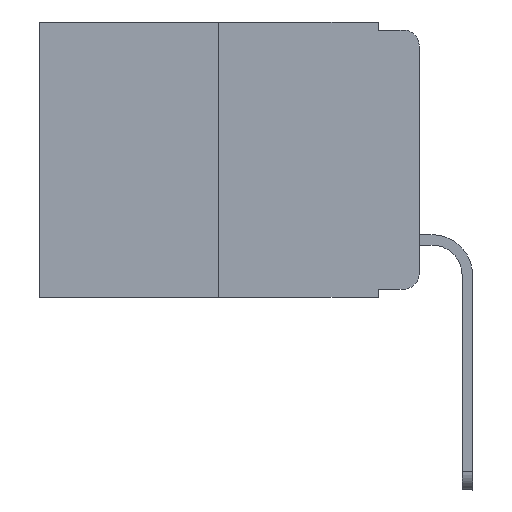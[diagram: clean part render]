
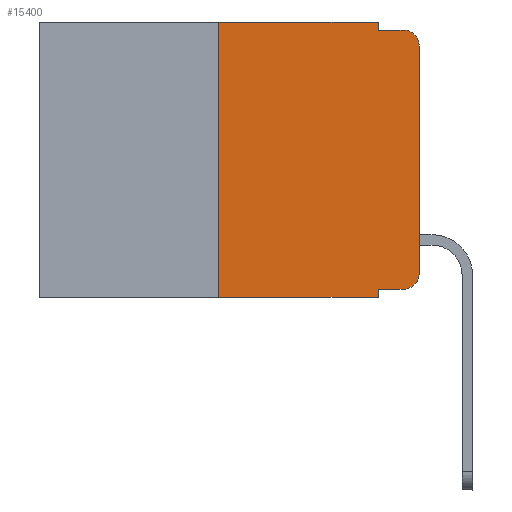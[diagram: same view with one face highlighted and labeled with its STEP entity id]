
A CAD part, left-side view. The second image highlights one B-rep face of the part: STEP entity #15400.
In plain terms, the highlighted planar face has unit normal (-1, 0, 0).
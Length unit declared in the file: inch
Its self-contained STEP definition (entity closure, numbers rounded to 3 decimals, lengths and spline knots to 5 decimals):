
#165 = VECTOR ( 'NONE', #6464, 39.37008 ) ;
#304 = EDGE_LOOP ( 'NONE', ( #10925, #14174, #7361, #12299, #2392, #10569, #844, #1517, #14218, #10826 ) ) ;
#573 = DIRECTION ( 'NONE',  ( 0., 0., 1. ) ) ;
#844 = ORIENTED_EDGE ( 'NONE', *, *, #16869, .T. ) ;
#1435 = CARTESIAN_POINT ( 'NONE',  ( 0., 0.051, 0. ) ) ;
#1517 = ORIENTED_EDGE ( 'NONE', *, *, #4754, .F. ) ;
#1707 = VECTOR ( 'NONE', #4496, 39.37008 ) ;
#1710 = DIRECTION ( 'NONE',  ( 1., 0., 0. ) ) ;
#2016 = LINE ( 'NONE', #16349, #14856 ) ;
#2392 = ORIENTED_EDGE ( 'NONE', *, *, #8061, .F. ) ;
#2592 = CARTESIAN_POINT ( 'NONE',  ( 0., 0.051, -0.01 ) ) ;
#2622 = LINE ( 'NONE', #18844, #1707 ) ;
#2809 = LINE ( 'NONE', #1435, #8584 ) ;
#2810 = CARTESIAN_POINT ( 'NONE',  ( 0., 0., -0.03 ) ) ;
#2931 = EDGE_CURVE ( 'NONE', #12350, #9406, #2622, .T. ) ;
#3103 = CIRCLE ( 'NONE', #6431, 0.02 ) ;
#3106 = CARTESIAN_POINT ( 'NONE',  ( 0., 0.051, -0.01 ) ) ;
#3170 = FACE_OUTER_BOUND ( 'NONE', #304, .T. ) ;
#3199 = VERTEX_POINT ( 'NONE', #14746 ) ;
#3351 = EDGE_CURVE ( 'NONE', #9406, #5729, #4566, .T. ) ;
#3366 = VERTEX_POINT ( 'NONE', #17032 ) ;
#3493 = CIRCLE ( 'NONE', #6182, 0.02 ) ;
#4496 = DIRECTION ( 'NONE',  ( 0., 0., -1. ) ) ;
#4566 = LINE ( 'NONE', #2592, #20115 ) ;
#4746 = LINE ( 'NONE', #6023, #20520 ) ;
#4754 = EDGE_CURVE ( 'NONE', #14351, #3199, #2809, .T. ) ;
#5729 = VERTEX_POINT ( 'NONE', #17383 ) ;
#5886 = DIRECTION ( 'NONE',  ( -1., 0., 0. ) ) ;
#6023 = CARTESIAN_POINT ( 'NONE',  ( 0., 0., 0. ) ) ;
#6074 = CARTESIAN_POINT ( 'NONE',  ( 0., 0.051, -0.333 ) ) ;
#6182 = AXIS2_PLACEMENT_3D ( 'NONE', #20226, #5886, #12489 ) ;
#6431 = AXIS2_PLACEMENT_3D ( 'NONE', #18303, #13614, #11941 ) ;
#6464 = DIRECTION ( 'NONE',  ( 0., -1., 0. ) ) ;
#7361 = ORIENTED_EDGE ( 'NONE', *, *, #3351, .F. ) ;
#7796 = CARTESIAN_POINT ( 'NONE',  ( 0., 0.051, 0. ) ) ;
#8061 = EDGE_CURVE ( 'NONE', #10872, #12350, #10120, .T. ) ;
#8144 = AXIS2_PLACEMENT_3D ( 'NONE', #8304, #1710, #17504 ) ;
#8304 = CARTESIAN_POINT ( 'NONE',  ( 0., 0.473, 0. ) ) ;
#8507 = VERTEX_POINT ( 'NONE', #9782 ) ;
#8584 = VECTOR ( 'NONE', #20389, 39.37008 ) ;
#8702 = EDGE_CURVE ( 'NONE', #14351, #11031, #2016, .T. ) ;
#9406 = VERTEX_POINT ( 'NONE', #3106 ) ;
#9612 = VECTOR ( 'NONE', #19637, 39.37008 ) ;
#9782 = CARTESIAN_POINT ( 'NONE',  ( 0., 0.25, -0.343 ) ) ;
#10120 = LINE ( 'NONE', #16487, #9612 ) ;
#10569 = ORIENTED_EDGE ( 'NONE', *, *, #20092, .F. ) ;
#10826 = ORIENTED_EDGE ( 'NONE', *, *, #14209, .T. ) ;
#10872 = VERTEX_POINT ( 'NONE', #15376 ) ;
#10925 = ORIENTED_EDGE ( 'NONE', *, *, #15254, .T. ) ;
#11031 = VERTEX_POINT ( 'NONE', #18348 ) ;
#11188 = LINE ( 'NONE', #17549, #165 ) ;
#11872 = DIRECTION ( 'NONE',  ( 0., -1., 0. ) ) ;
#11941 = DIRECTION ( 'NONE',  ( 0., 0., -1. ) ) ;
#12007 = VECTOR ( 'NONE', #573, 39.37008 ) ;
#12299 = ORIENTED_EDGE ( 'NONE', *, *, #2931, .F. ) ;
#12350 = VERTEX_POINT ( 'NONE', #7796 ) ;
#12489 = DIRECTION ( 'NONE',  ( 0., 0., -1. ) ) ;
#13614 = DIRECTION ( 'NONE',  ( -1., 0., 0. ) ) ;
#13811 = DIRECTION ( 'NONE',  ( 0., -1., 0. ) ) ;
#14174 = ORIENTED_EDGE ( 'NONE', *, *, #16227, .T. ) ;
#14209 = EDGE_CURVE ( 'NONE', #11031, #3366, #3103, .T. ) ;
#14218 = ORIENTED_EDGE ( 'NONE', *, *, #8702, .T. ) ;
#14351 = VERTEX_POINT ( 'NONE', #6074 ) ;
#14379 = PLANE ( 'NONE',  #8144 ) ;
#14718 = CARTESIAN_POINT ( 'NONE',  ( 0., 0.25, 0. ) ) ;
#14746 = CARTESIAN_POINT ( 'NONE',  ( 0., 0.051, -0.343 ) ) ;
#14856 = VECTOR ( 'NONE', #11872, 39.37008 ) ;
#14915 = LINE ( 'NONE', #14718, #12007 ) ;
#15254 = EDGE_CURVE ( 'NONE', #3366, #19811, #4746, .T. ) ;
#15376 = CARTESIAN_POINT ( 'NONE',  ( 0., 0.25, 0. ) ) ;
#15400 = ADVANCED_FACE ( 'NONE', ( #3170 ), #14379, .F. ) ;
#16227 = EDGE_CURVE ( 'NONE', #19811, #5729, #3493, .T. ) ;
#16349 = CARTESIAN_POINT ( 'NONE',  ( 0., 0.051, -0.333 ) ) ;
#16487 = CARTESIAN_POINT ( 'NONE',  ( 0., 0.473, 0. ) ) ;
#16869 = EDGE_CURVE ( 'NONE', #8507, #3199, #11188, .T. ) ;
#17001 = DIRECTION ( 'NONE',  ( 0., 0., 1. ) ) ;
#17032 = CARTESIAN_POINT ( 'NONE',  ( 0., 0., -0.313 ) ) ;
#17383 = CARTESIAN_POINT ( 'NONE',  ( 0., 0.02, -0.01 ) ) ;
#17504 = DIRECTION ( 'NONE',  ( 0., 0., -1. ) ) ;
#17549 = CARTESIAN_POINT ( 'NONE',  ( 0., 0.473, -0.343 ) ) ;
#18303 = CARTESIAN_POINT ( 'NONE',  ( 0., 0.02, -0.313 ) ) ;
#18348 = CARTESIAN_POINT ( 'NONE',  ( 0., 0.02, -0.333 ) ) ;
#18844 = CARTESIAN_POINT ( 'NONE',  ( 0., 0.051, 0. ) ) ;
#19637 = DIRECTION ( 'NONE',  ( 0., -1., 0. ) ) ;
#19811 = VERTEX_POINT ( 'NONE', #2810 ) ;
#20092 = EDGE_CURVE ( 'NONE', #8507, #10872, #14915, .T. ) ;
#20115 = VECTOR ( 'NONE', #13811, 39.37008 ) ;
#20226 = CARTESIAN_POINT ( 'NONE',  ( 0., 0.02, -0.03 ) ) ;
#20389 = DIRECTION ( 'NONE',  ( 0., 0., -1. ) ) ;
#20520 = VECTOR ( 'NONE', #17001, 39.37008 ) ;
